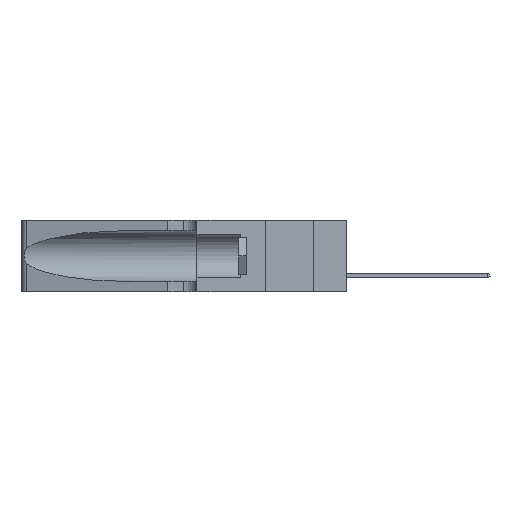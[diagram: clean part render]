
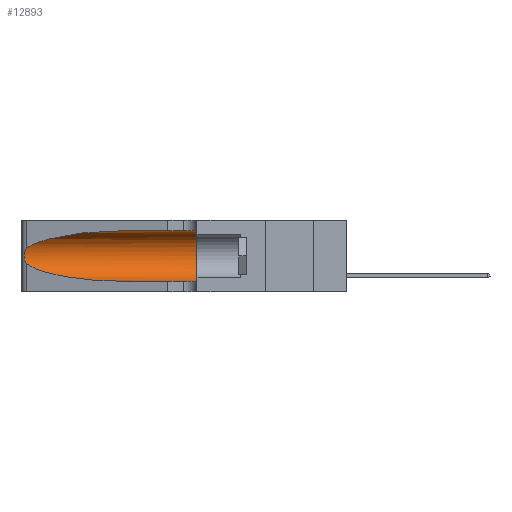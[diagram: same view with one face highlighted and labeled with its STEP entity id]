
A CAD part, left-side view. The second image highlights one B-rep face of the part: STEP entity #12893.
In plain terms, the highlighted cylindrical face has radius 3.308 mm (diameter 6.617 mm), a partial arc.
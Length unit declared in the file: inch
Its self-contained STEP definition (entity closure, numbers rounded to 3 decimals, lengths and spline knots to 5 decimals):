
#32 = VERTEX_POINT ( 'NONE', #14862 ) ;
#1796 = CARTESIAN_POINT ( 'NONE',  ( 0.1305, 0.72297, 0.31525 ) ) ;
#2319 = CARTESIAN_POINT ( 'NONE',  ( 0.25487, 1.22718, 0.22369 ) ) ;
#2421 = DIRECTION ( 'NONE',  ( 0., -1., 0. ) ) ;
#2558 = CARTESIAN_POINT ( 'NONE',  ( 0.25787, 1.23484, 0.2124 ) ) ;
#3665 = VERTEX_POINT ( 'NONE', #22625 ) ;
#3744 = CARTESIAN_POINT ( 'NONE',  ( 0.25854, 1.2359, 0.20912 ) ) ;
#8389 = CARTESIAN_POINT ( 'NONE',  ( 0.25487, 1.22718, 0.22369 ) ) ;
#9697 = CIRCLE ( 'NONE', #30689, 0.13025 ) ;
#10419 = ORIENTED_EDGE ( 'NONE', *, *, #40860, .F. ) ;
#11441 = CARTESIAN_POINT ( 'NONE',  ( 0.26075, 1.23896, 0.178 ) ) ;
#12893 = ADVANCED_FACE ( 'NONE', ( #33323 ), #40088, .F. ) ;
#13616 = AXIS2_PLACEMENT_3D ( 'NONE', #19556, #34565, #35957 ) ;
#14862 = CARTESIAN_POINT ( 'NONE',  ( 0.1305, 0.35, 0.31525 ) ) ;
#15185 = CARTESIAN_POINT ( 'NONE',  ( 0.26018, 1.23835, 0.19895 ) ) ;
#16214 = CARTESIAN_POINT ( 'NONE',  ( 0.25856, 1.23593, 0.16098 ) ) ;
#16930 = ORIENTED_EDGE ( 'NONE', *, *, #31282, .T. ) ;
#17491 = CARTESIAN_POINT ( 'NONE',  ( 0.25487, 1.22718, 0.14631 ) ) ;
#17599 = CARTESIAN_POINT ( 'NONE',  ( 0.25487, 1.22718, 0.14631 ) ) ;
#18042 = CARTESIAN_POINT ( 'NONE',  ( 0.2373, 1.15595, 0.28018 ) ) ;
#18171 = VERTEX_POINT ( 'NONE', #17491 ) ;
#18834 = DIRECTION ( 'NONE',  ( 0., 0., 1. ) ) ;
#19556 = CARTESIAN_POINT ( 'NONE',  ( 0.1305, 1.61858, 0.185 ) ) ;
#19971 = CARTESIAN_POINT ( 'NONE',  ( 0.25639, 1.23186, 0.15144 ) ) ;
#20144 = CARTESIAN_POINT ( 'NONE',  ( 0.25555, 1.22993, 0.14849 ) ) ;
#20328 = EDGE_CURVE ( 'NONE', #29281, #18171, #22381, .T. ) ;
#20542 = VECTOR ( 'NONE', #2421, 39.37008 ) ;
#21136 = CARTESIAN_POINT ( 'NONE',  ( 0.18966, 0.96281, 0.31525 ) ) ;
#21195 = VERTEX_POINT ( 'NONE', #35201 ) ;
#22381 = B_SPLINE_CURVE_WITH_KNOTS ( 'NONE', 3,
 ( #29675, #37930, #33620, #2558, #3744, #15185, #30894, #11441, #31235, #16214, #32053, #19971, #20144, #36514 ),
 .UNSPECIFIED., .F., .F.,
 ( 4, 2, 2, 2, 2, 2, 4 ),
 ( 0., 0.00027, 0.00053, 0.00107, 0.0016, 0.00187, 0.00214 ),
 .UNSPECIFIED. ) ;
#22625 = CARTESIAN_POINT ( 'NONE',  ( 0.1305, 0.35, 0.05475 ) ) ;
#23028 =( BOUNDED_CURVE ( )  B_SPLINE_CURVE ( 3, ( #17599, #45440, #48858, #29499 ),
 .UNSPECIFIED., .F., .T. ) 
 B_SPLINE_CURVE_WITH_KNOTS ( ( 4, 4 ),
 ( 3.44316, 4.71239 ),
 .UNSPECIFIED. ) 
 CURVE ( )  GEOMETRIC_REPRESENTATION_ITEM ( )  RATIONAL_B_SPLINE_CURVE ( ( 1., 0.87, 0.87, 1. ) ) 
 REPRESENTATION_ITEM ( '' )  );
#23608 = ORIENTED_EDGE ( 'NONE', *, *, #20328, .T. ) ;
#25009 = EDGE_CURVE ( 'NONE', #32, #3665, #9697, .T. ) ;
#25945 = EDGE_CURVE ( 'NONE', #21195, #3665, #44414, .T. ) ;
#26109 =( BOUNDED_CURVE ( )  B_SPLINE_CURVE ( 3, ( #40108, #21136, #18042, #2319 ),
 .UNSPECIFIED., .F., .F. ) 
 B_SPLINE_CURVE_WITH_KNOTS ( ( 4, 4 ),
 ( 1.5708, 2.84003 ),
 .UNSPECIFIED. ) 
 CURVE ( )  GEOMETRIC_REPRESENTATION_ITEM ( )  RATIONAL_B_SPLINE_CURVE ( ( 1., 0.87, 0.87, 1. ) ) 
 REPRESENTATION_ITEM ( '' )  );
#29281 = VERTEX_POINT ( 'NONE', #8389 ) ;
#29499 = CARTESIAN_POINT ( 'NONE',  ( 0.1305, 0.72297, 0.05475 ) ) ;
#29675 = CARTESIAN_POINT ( 'NONE',  ( 0.25487, 1.22718, 0.22369 ) ) ;
#30412 = DIRECTION ( 'NONE',  ( 0., 1., 0. ) ) ;
#30689 = AXIS2_PLACEMENT_3D ( 'NONE', #46662, #30412, #18834 ) ;
#30894 = CARTESIAN_POINT ( 'NONE',  ( 0.26075, 1.23896, 0.19203 ) ) ;
#31053 = CARTESIAN_POINT ( 'NONE',  ( 0.1305, 1.61858, 0.05475 ) ) ;
#31235 = CARTESIAN_POINT ( 'NONE',  ( 0.26017, 1.23833, 0.17102 ) ) ;
#31282 = EDGE_CURVE ( 'NONE', #18171, #21195, #23028, .T. ) ;
#32053 = CARTESIAN_POINT ( 'NONE',  ( 0.25789, 1.23486, 0.15765 ) ) ;
#32919 = ORIENTED_EDGE ( 'NONE', *, *, #25945, .T. ) ;
#33323 = FACE_OUTER_BOUND ( 'NONE', #44058, .T. ) ;
#33620 = CARTESIAN_POINT ( 'NONE',  ( 0.25639, 1.23184, 0.21858 ) ) ;
#34262 = ORIENTED_EDGE ( 'NONE', *, *, #25009, .F. ) ;
#34565 = DIRECTION ( 'NONE',  ( 0., -1., 0. ) ) ;
#34860 = EDGE_CURVE ( 'NONE', #39009, #29281, #26109, .T. ) ;
#35201 = CARTESIAN_POINT ( 'NONE',  ( 0.1305, 0.72297, 0.05475 ) ) ;
#35957 = DIRECTION ( 'NONE',  ( 0., 0., -1. ) ) ;
#36430 = LINE ( 'NONE', #39869, #20542 ) ;
#36514 = CARTESIAN_POINT ( 'NONE',  ( 0.25487, 1.22718, 0.14631 ) ) ;
#37930 = CARTESIAN_POINT ( 'NONE',  ( 0.25555, 1.22994, 0.2215 ) ) ;
#39009 = VERTEX_POINT ( 'NONE', #1796 ) ;
#39869 = CARTESIAN_POINT ( 'NONE',  ( 0.1305, 1.61858, 0.31525 ) ) ;
#40088 = CYLINDRICAL_SURFACE ( 'NONE', #13616, 0.13025 ) ;
#40108 = CARTESIAN_POINT ( 'NONE',  ( 0.1305, 0.72297, 0.31525 ) ) ;
#40860 = EDGE_CURVE ( 'NONE', #39009, #32, #36430, .T. ) ;
#41644 = ORIENTED_EDGE ( 'NONE', *, *, #34860, .T. ) ;
#43206 = DIRECTION ( 'NONE',  ( 0., -1., 0. ) ) ;
#44058 = EDGE_LOOP ( 'NONE', ( #41644, #23608, #16930, #32919, #34262, #10419 ) ) ;
#44414 = LINE ( 'NONE', #31053, #48084 ) ;
#45440 = CARTESIAN_POINT ( 'NONE',  ( 0.2373, 1.15595, 0.08982 ) ) ;
#46662 = CARTESIAN_POINT ( 'NONE',  ( 0.1305, 0.35, 0.185 ) ) ;
#48084 = VECTOR ( 'NONE', #43206, 39.37008 ) ;
#48858 = CARTESIAN_POINT ( 'NONE',  ( 0.18966, 0.96281, 0.05475 ) ) ;
